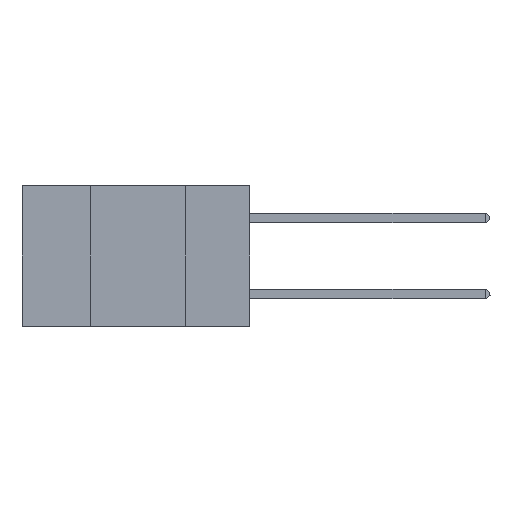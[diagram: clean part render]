
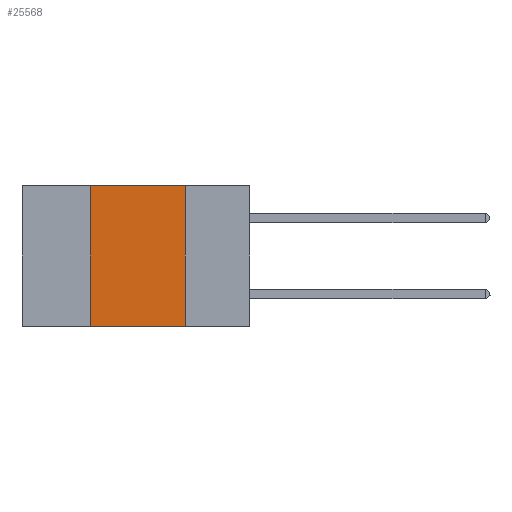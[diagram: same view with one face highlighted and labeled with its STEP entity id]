
A CAD part, left-side view. The second image highlights one B-rep face of the part: STEP entity #25568.
In plain terms, the highlighted planar face has unit normal (-1, 0, 0).
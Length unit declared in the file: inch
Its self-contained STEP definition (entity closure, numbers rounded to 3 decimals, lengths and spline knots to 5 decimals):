
#4813 = CARTESIAN_POINT ( 'NONE',  ( 0., 0.6, 0. ) ) ;
#5278 = VERTEX_POINT ( 'NONE', #30519 ) ;
#6454 = ORIENTED_EDGE ( 'NONE', *, *, #23659, .F. ) ;
#6855 = CARTESIAN_POINT ( 'NONE',  ( 0., 0.6, -0.37 ) ) ;
#6939 = LINE ( 'NONE', #10901, #13072 ) ;
#7835 = CARTESIAN_POINT ( 'NONE',  ( 0., 0.17, 0. ) ) ;
#8135 = CARTESIAN_POINT ( 'NONE',  ( 0., 0.42, 0. ) ) ;
#8511 = CARTESIAN_POINT ( 'NONE',  ( 0., 0.6, 0. ) ) ;
#9859 = DIRECTION ( 'NONE',  ( 1., 0., 0. ) ) ;
#10140 = VECTOR ( 'NONE', #18073, 39.37008 ) ;
#10901 = CARTESIAN_POINT ( 'NONE',  ( 0., 0.42, 0. ) ) ;
#11251 = DIRECTION ( 'NONE',  ( 0., -1., 0. ) ) ;
#11554 = AXIS2_PLACEMENT_3D ( 'NONE', #4813, #9859, #28263 ) ;
#11686 = ORIENTED_EDGE ( 'NONE', *, *, #11816, .F. ) ;
#11816 = EDGE_CURVE ( 'NONE', #5278, #12764, #6939, .T. ) ;
#12395 = LINE ( 'NONE', #8511, #24994 ) ;
#12599 = PLANE ( 'NONE',  #11554 ) ;
#12764 = VERTEX_POINT ( 'NONE', #8135 ) ;
#13072 = VECTOR ( 'NONE', #31722, 39.37008 ) ;
#15051 = DIRECTION ( 'NONE',  ( 0., -1., 0. ) ) ;
#15216 = FACE_OUTER_BOUND ( 'NONE', #32177, .T. ) ;
#16383 = LINE ( 'NONE', #6855, #28595 ) ;
#17039 = LINE ( 'NONE', #7835, #10140 ) ;
#17614 = ORIENTED_EDGE ( 'NONE', *, *, #25134, .F. ) ;
#17629 = CARTESIAN_POINT ( 'NONE',  ( 0., 0.17, -0.37 ) ) ;
#18073 = DIRECTION ( 'NONE',  ( 0., 0., -1. ) ) ;
#19360 = VERTEX_POINT ( 'NONE', #24290 ) ;
#23659 = EDGE_CURVE ( 'NONE', #19360, #26884, #17039, .T. ) ;
#24290 = CARTESIAN_POINT ( 'NONE',  ( 0., 0.17, 0. ) ) ;
#24994 = VECTOR ( 'NONE', #11251, 39.37008 ) ;
#25134 = EDGE_CURVE ( 'NONE', #12764, #19360, #12395, .T. ) ;
#25523 = ORIENTED_EDGE ( 'NONE', *, *, #26183, .T. ) ;
#25568 = ADVANCED_FACE ( 'NONE', ( #15216 ), #12599, .F. ) ;
#26183 = EDGE_CURVE ( 'NONE', #5278, #26884, #16383, .T. ) ;
#26884 = VERTEX_POINT ( 'NONE', #17629 ) ;
#28263 = DIRECTION ( 'NONE',  ( 0., 0., -1. ) ) ;
#28595 = VECTOR ( 'NONE', #15051, 39.37008 ) ;
#30519 = CARTESIAN_POINT ( 'NONE',  ( 0., 0.42, -0.37 ) ) ;
#31722 = DIRECTION ( 'NONE',  ( 0., 0., 1. ) ) ;
#32177 = EDGE_LOOP ( 'NONE', ( #6454, #17614, #11686, #25523 ) ) ;
